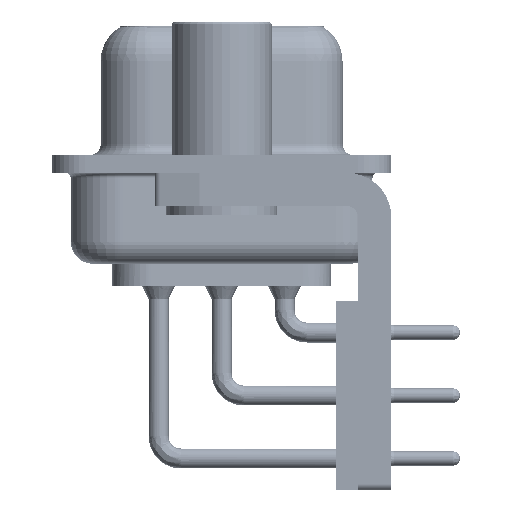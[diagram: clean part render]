
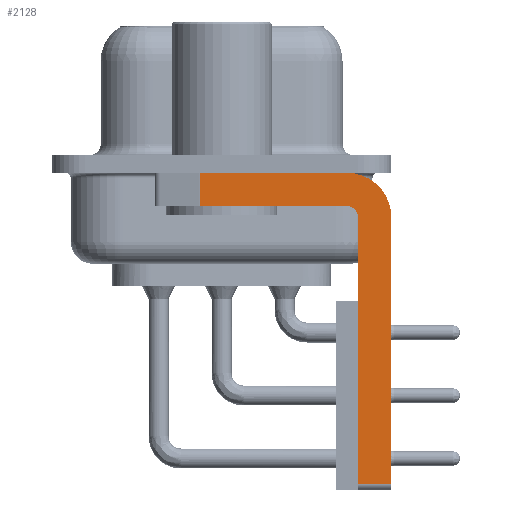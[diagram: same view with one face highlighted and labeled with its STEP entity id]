
A CAD part, left-side view. The second image highlights one B-rep face of the part: STEP entity #2128.
In plain terms, the highlighted planar face has unit normal (-1, 0, 0).
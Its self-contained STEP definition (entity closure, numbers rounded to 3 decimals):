
#632 = CARTESIAN_POINT ( 'NONE',  ( -2.9, -5.65, -14.45 ) ) ;
#717 = VERTEX_POINT ( 'NONE', #26148 ) ;
#2030 = DIRECTION ( 'NONE',  ( 0., 0., -1. ) ) ;
#2128 = ADVANCED_FACE ( 'NONE', ( #30880 ), #37221, .F. ) ;
#2386 = VERTEX_POINT ( 'NONE', #30892 ) ;
#3112 = VECTOR ( 'NONE', #37547, 1000. ) ;
#4090 = VERTEX_POINT ( 'NONE', #35954 ) ;
#4718 = CARTESIAN_POINT ( 'NONE',  ( -2.9, 0.978, -1.9 ) ) ;
#5668 = EDGE_CURVE ( 'NONE', #717, #4090, #26536, .T. ) ;
#6200 = CARTESIAN_POINT ( 'NONE',  ( -2.9, -5.65, -1.9 ) ) ;
#6289 = AXIS2_PLACEMENT_3D ( 'NONE', #34622, #34499, #35739 ) ;
#8130 = LINE ( 'NONE', #632, #38231 ) ;
#9286 = CARTESIAN_POINT ( 'NONE',  ( -2.9, -5.65, -2.4 ) ) ;
#9313 = EDGE_CURVE ( 'NONE', #24739, #24778, #30948, .T. ) ;
#10308 = LINE ( 'NONE', #29910, #32251 ) ;
#10645 = EDGE_CURVE ( 'NONE', #24778, #26071, #10308, .T. ) ;
#10676 = CARTESIAN_POINT ( 'NONE',  ( -2.9, -6.15, -14.7 ) ) ;
#11175 = LINE ( 'NONE', #17437, #34036 ) ;
#11329 = AXIS2_PLACEMENT_3D ( 'NONE', #38874, #38701, #38654 ) ;
#11920 = DIRECTION ( 'NONE',  ( 0., 1., 0. ) ) ;
#12355 = DIRECTION ( 'NONE',  ( 0., 0., 1. ) ) ;
#12562 = DIRECTION ( 'NONE',  ( 0., -1., 0. ) ) ;
#12915 = DIRECTION ( 'NONE',  ( 0., 0., -1. ) ) ;
#14710 = LINE ( 'NONE', #33769, #37711 ) ;
#15090 = EDGE_CURVE ( 'NONE', #4090, #29230, #14710, .T. ) ;
#15556 = ORIENTED_EDGE ( 'NONE', *, *, #10645, .F. ) ;
#15860 = VECTOR ( 'NONE', #12562, 1000. ) ;
#16220 = ORIENTED_EDGE ( 'NONE', *, *, #15090, .F. ) ;
#16253 = EDGE_CURVE ( 'NONE', #37895, #29230, #8130, .T. ) ;
#17437 = CARTESIAN_POINT ( 'NONE',  ( -2.9, 0.978, -1.9 ) ) ;
#18310 = CARTESIAN_POINT ( 'NONE',  ( -2.9, -6.15, -14.45 ) ) ;
#19375 = LINE ( 'NONE', #10676, #3112 ) ;
#21404 = EDGE_LOOP ( 'NONE', ( #21733, #33808, #15556, #33732, #29989, #22761, #16220, #39158 ) ) ;
#21733 = ORIENTED_EDGE ( 'NONE', *, *, #28087, .F. ) ;
#22761 = ORIENTED_EDGE ( 'NONE', *, *, #16253, .T. ) ;
#23831 = LINE ( 'NONE', #30421, #15860 ) ;
#24739 = VERTEX_POINT ( 'NONE', #39001 ) ;
#24778 = VERTEX_POINT ( 'NONE', #6200 ) ;
#24952 = AXIS2_PLACEMENT_3D ( 'NONE', #9286, #30213, #12355 ) ;
#26071 = VERTEX_POINT ( 'NONE', #4718 ) ;
#26148 = CARTESIAN_POINT ( 'NONE',  ( -2.9, -5.65, -0.4 ) ) ;
#26536 = CIRCLE ( 'NONE', #11329, 2. ) ;
#28087 = EDGE_CURVE ( 'NONE', #2386, #717, #23831, .T. ) ;
#28479 = CARTESIAN_POINT ( 'NONE',  ( -2.9, -7.65, -14.45 ) ) ;
#29230 = VERTEX_POINT ( 'NONE', #28479 ) ;
#29910 = CARTESIAN_POINT ( 'NONE',  ( -2.9, -5.65, -1.9 ) ) ;
#29989 = ORIENTED_EDGE ( 'NONE', *, *, #32852, .F. ) ;
#30213 = DIRECTION ( 'NONE',  ( -1., 0., 0. ) ) ;
#30421 = CARTESIAN_POINT ( 'NONE',  ( -2.9, 3., -0.4 ) ) ;
#30813 = DIRECTION ( 'NONE',  ( 0., -1., 0. ) ) ;
#30880 = FACE_OUTER_BOUND ( 'NONE', #21404, .T. ) ;
#30892 = CARTESIAN_POINT ( 'NONE',  ( -2.9, 0.978, -0.4 ) ) ;
#30948 = CIRCLE ( 'NONE', #24952, 0.5 ) ;
#32251 = VECTOR ( 'NONE', #11920, 1000. ) ;
#32852 = EDGE_CURVE ( 'NONE', #37895, #24739, #19375, .T. ) ;
#33732 = ORIENTED_EDGE ( 'NONE', *, *, #9313, .F. ) ;
#33769 = CARTESIAN_POINT ( 'NONE',  ( -2.9, -7.65, -2.4 ) ) ;
#33808 = ORIENTED_EDGE ( 'NONE', *, *, #37049, .T. ) ;
#34036 = VECTOR ( 'NONE', #2030, 1000. ) ;
#34499 = DIRECTION ( 'NONE',  ( 1., 0., 0. ) ) ;
#34622 = CARTESIAN_POINT ( 'NONE',  ( -2.9, -5.65, -2.4 ) ) ;
#35739 = DIRECTION ( 'NONE',  ( 0., 0., -1. ) ) ;
#35954 = CARTESIAN_POINT ( 'NONE',  ( -2.9, -7.65, -2.4 ) ) ;
#37049 = EDGE_CURVE ( 'NONE', #2386, #26071, #11175, .T. ) ;
#37221 = PLANE ( 'NONE',  #6289 ) ;
#37547 = DIRECTION ( 'NONE',  ( 0., 0., 1. ) ) ;
#37711 = VECTOR ( 'NONE', #12915, 1000. ) ;
#37895 = VERTEX_POINT ( 'NONE', #18310 ) ;
#38231 = VECTOR ( 'NONE', #30813, 1000. ) ;
#38654 = DIRECTION ( 'NONE',  ( 0., 0., -1. ) ) ;
#38701 = DIRECTION ( 'NONE',  ( 1., 0., 0. ) ) ;
#38874 = CARTESIAN_POINT ( 'NONE',  ( -2.9, -5.65, -2.4 ) ) ;
#39001 = CARTESIAN_POINT ( 'NONE',  ( -2.9, -6.15, -2.4 ) ) ;
#39158 = ORIENTED_EDGE ( 'NONE', *, *, #5668, .F. ) ;
